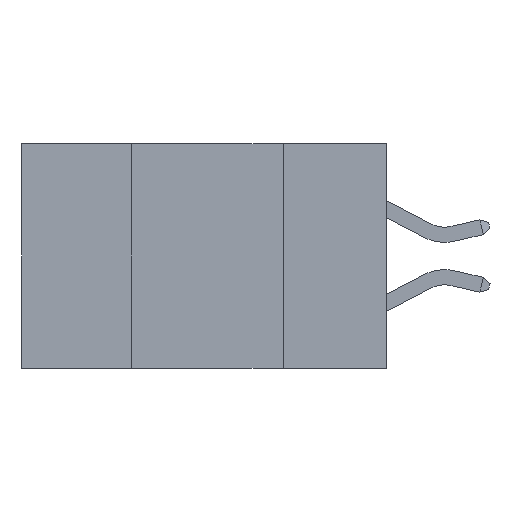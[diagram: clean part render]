
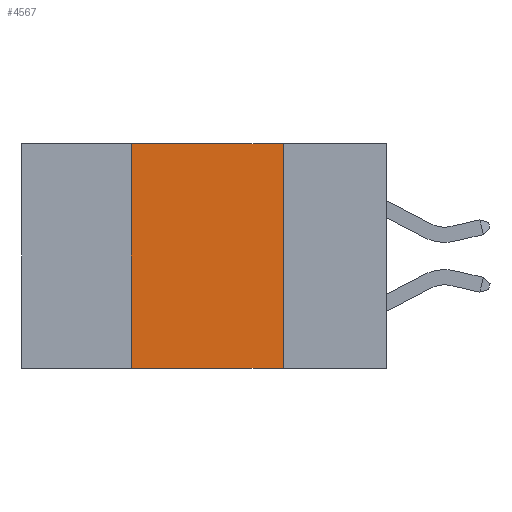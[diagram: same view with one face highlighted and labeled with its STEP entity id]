
A CAD part, left-side view. The second image highlights one B-rep face of the part: STEP entity #4567.
In plain terms, the highlighted planar face has unit normal (-1, 0, 0).
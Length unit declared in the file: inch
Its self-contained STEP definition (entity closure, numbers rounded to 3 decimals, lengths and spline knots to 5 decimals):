
#581 = VECTOR ( 'NONE', #8154, 39.37008 ) ;
#1018 = ORIENTED_EDGE ( 'NONE', *, *, #4931, .F. ) ;
#1400 = ORIENTED_EDGE ( 'NONE', *, *, #6386, .F. ) ;
#1498 = EDGE_CURVE ( 'NONE', #9589, #7534, #8758, .T. ) ;
#1711 = LINE ( 'NONE', #3036, #2848 ) ;
#2460 = EDGE_LOOP ( 'NONE', ( #1400, #6628, #1018, #8237 ) ) ;
#2848 = VECTOR ( 'NONE', #8812, 39.37008 ) ;
#3036 = CARTESIAN_POINT ( 'NONE',  ( 0., 0.42, 0. ) ) ;
#3320 = CARTESIAN_POINT ( 'NONE',  ( 0., 0.42, 0. ) ) ;
#3408 = VECTOR ( 'NONE', #3866, 39.37008 ) ;
#3835 = DIRECTION ( 'NONE',  ( 0., 0., -1. ) ) ;
#3866 = DIRECTION ( 'NONE',  ( 0., -1., 0. ) ) ;
#3915 = CARTESIAN_POINT ( 'NONE',  ( 0., 0.6, 0. ) ) ;
#4311 = LINE ( 'NONE', #4692, #3408 ) ;
#4505 = LINE ( 'NONE', #7393, #581 ) ;
#4567 = ADVANCED_FACE ( 'NONE', ( #5631 ), #10563, .F. ) ;
#4692 = CARTESIAN_POINT ( 'NONE',  ( 0., 0.6, 0. ) ) ;
#4903 = DIRECTION ( 'NONE',  ( 0., -1., 0. ) ) ;
#4931 = EDGE_CURVE ( 'NONE', #9589, #6142, #1711, .T. ) ;
#5567 = DIRECTION ( 'NONE',  ( 1., 0., 0. ) ) ;
#5631 = FACE_OUTER_BOUND ( 'NONE', #2460, .T. ) ;
#6142 = VERTEX_POINT ( 'NONE', #3320 ) ;
#6347 = AXIS2_PLACEMENT_3D ( 'NONE', #3915, #5567, #3835 ) ;
#6386 = EDGE_CURVE ( 'NONE', #10612, #7534, #4505, .T. ) ;
#6628 = ORIENTED_EDGE ( 'NONE', *, *, #10737, .F. ) ;
#7393 = CARTESIAN_POINT ( 'NONE',  ( 0., 0.17, 0. ) ) ;
#7394 = CARTESIAN_POINT ( 'NONE',  ( 0., 0.6, -0.37 ) ) ;
#7534 = VERTEX_POINT ( 'NONE', #10683 ) ;
#7997 = CARTESIAN_POINT ( 'NONE',  ( 0., 0.17, 0. ) ) ;
#7998 = CARTESIAN_POINT ( 'NONE',  ( 0., 0.42, -0.37 ) ) ;
#8154 = DIRECTION ( 'NONE',  ( 0., 0., -1. ) ) ;
#8237 = ORIENTED_EDGE ( 'NONE', *, *, #1498, .T. ) ;
#8358 = VECTOR ( 'NONE', #4903, 39.37008 ) ;
#8758 = LINE ( 'NONE', #7394, #8358 ) ;
#8812 = DIRECTION ( 'NONE',  ( 0., 0., 1. ) ) ;
#9589 = VERTEX_POINT ( 'NONE', #7998 ) ;
#10563 = PLANE ( 'NONE',  #6347 ) ;
#10612 = VERTEX_POINT ( 'NONE', #7997 ) ;
#10683 = CARTESIAN_POINT ( 'NONE',  ( 0., 0.17, -0.37 ) ) ;
#10737 = EDGE_CURVE ( 'NONE', #6142, #10612, #4311, .T. ) ;
